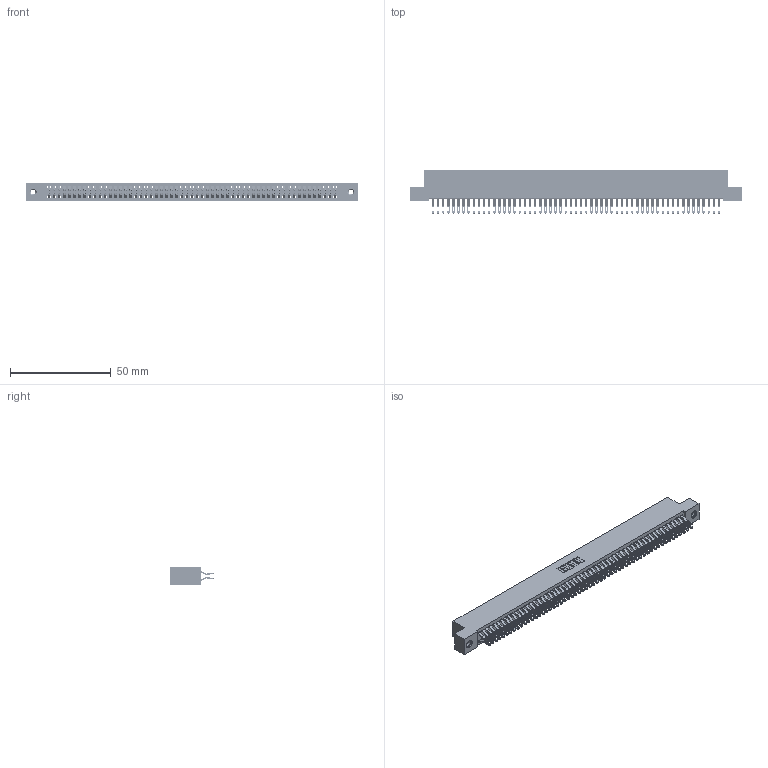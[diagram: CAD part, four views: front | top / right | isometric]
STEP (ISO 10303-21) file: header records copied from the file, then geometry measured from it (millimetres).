
FILE_DESCRIPTION (( 'STEP AP203' ), '1' );
FILE_NAME ('392-114-555-208.STEP', '2019-10-10T01:14:56', ( '' ), ( '' ), 'SwSTEP 2.0', 'SolidWorks 2016', '' );
FILE_SCHEMA (( 'CONFIG_CONTROL_DESIGN' ));
Length unit declared in the file: inch
Products named in the file (4): 342 Part_TI; 345-292-001_555 Tail; 345-250-001_345-250-003-102; 392-114-555-208
Assembly tree (117 placements, depth 2):
  392-114-555-208
    342 Part_TI
    345-292-001_555 Tail  x114
    345-250-001_345-250-003-102  x2
Bounding box: 165.1 x 21.47 x 9.4 mm (x, y, z)
Volume: 15216.3 mm3; surface area: 26251.3 mm2
Topology: 117 solids, 117 shells, 6782 faces, 21297 edges, 14190 vertices
Faces by surface type: plane 3974, cylinder 2792, cone 12, torus 4
Entity records: 36110 total; most frequent: CARTESIAN_POINT 5983, ORIENTED_EDGE 5882, DIRECTION 5087, EDGE_CURVE 2941, LINE 2773, VECTOR 2773, VERTEX_POINT 1956, AXIS2_PLACEMENT_3D 1157
